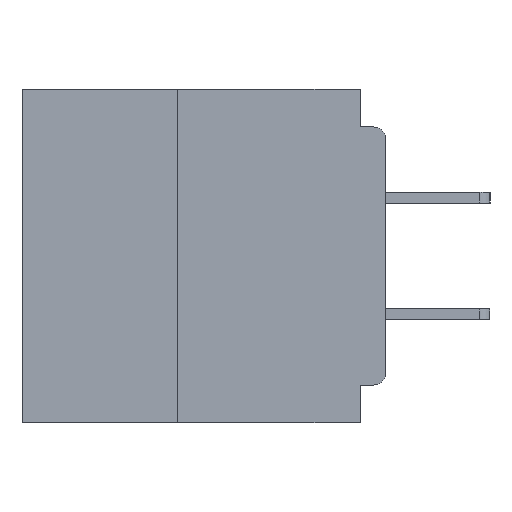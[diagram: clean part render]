
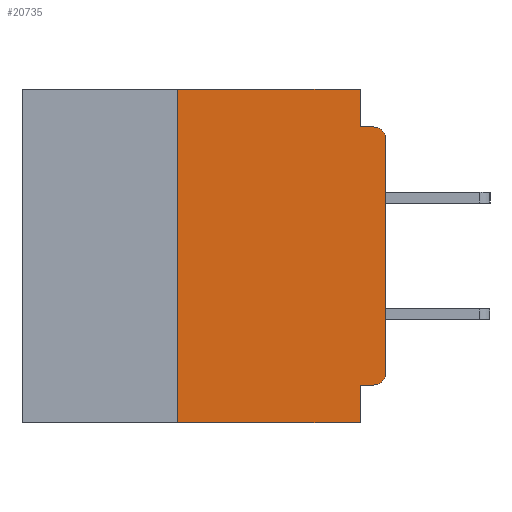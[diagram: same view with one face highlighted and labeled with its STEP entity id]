
A CAD part, left-side view. The second image highlights one B-rep face of the part: STEP entity #20735.
In plain terms, the highlighted planar face has unit normal (-1, 0, 0).
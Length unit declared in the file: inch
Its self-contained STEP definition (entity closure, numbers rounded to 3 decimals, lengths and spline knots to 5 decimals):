
#70 = VECTOR ( 'NONE', #9603, 39.37008 ) ;
#763 = ORIENTED_EDGE ( 'NONE', *, *, #41111, .F. ) ;
#1189 = AXIS2_PLACEMENT_3D ( 'NONE', #9205, #21796, #34524 ) ;
#1302 = ORIENTED_EDGE ( 'NONE', *, *, #34901, .T. ) ;
#3317 = LINE ( 'NONE', #16609, #27731 ) ;
#3838 = CARTESIAN_POINT ( 'NONE',  ( 0., 0.25, -0.4 ) ) ;
#3879 = VERTEX_POINT ( 'NONE', #12400 ) ;
#4194 = DIRECTION ( 'NONE',  ( 0., 0., -1. ) ) ;
#4347 = DIRECTION ( 'NONE',  ( 0., 0., -1. ) ) ;
#4814 = ORIENTED_EDGE ( 'NONE', *, *, #25874, .F. ) ;
#5164 = DIRECTION ( 'NONE',  ( 0., -1., 0. ) ) ;
#6612 = VERTEX_POINT ( 'NONE', #13823 ) ;
#7369 = ORIENTED_EDGE ( 'NONE', *, *, #7548, .T. ) ;
#7548 = EDGE_CURVE ( 'NONE', #29300, #3879, #25821, .T. ) ;
#7783 = VERTEX_POINT ( 'NONE', #19873 ) ;
#8042 = CARTESIAN_POINT ( 'NONE',  ( 0., 0.031, -0.045 ) ) ;
#8632 = CARTESIAN_POINT ( 'NONE',  ( 0., 0.015, -0.045 ) ) ;
#8932 = VECTOR ( 'NONE', #26107, 39.37008 ) ;
#9205 = CARTESIAN_POINT ( 'NONE',  ( 0., 0.437, 0. ) ) ;
#9603 = DIRECTION ( 'NONE',  ( 0., -1., 0. ) ) ;
#10571 = LINE ( 'NONE', #23249, #26465 ) ;
#12393 = PLANE ( 'NONE',  #1189 ) ;
#12400 = CARTESIAN_POINT ( 'NONE',  ( 0., 0., -0.34 ) ) ;
#12407 = LINE ( 'NONE', #19361, #30277 ) ;
#13121 = VERTEX_POINT ( 'NONE', #8042 ) ;
#13267 = VERTEX_POINT ( 'NONE', #15220 ) ;
#13597 = EDGE_CURVE ( 'NONE', #13267, #25910, #10571, .T. ) ;
#13823 = CARTESIAN_POINT ( 'NONE',  ( 0., 0.031, 0. ) ) ;
#13859 = LINE ( 'NONE', #23425, #38057 ) ;
#14188 = LINE ( 'NONE', #21141, #30055 ) ;
#14598 = VECTOR ( 'NONE', #20592, 39.37008 ) ;
#15053 = CARTESIAN_POINT ( 'NONE',  ( 0., 0.031, -0.4 ) ) ;
#15114 = AXIS2_PLACEMENT_3D ( 'NONE', #34560, #15597, #37705 ) ;
#15220 = CARTESIAN_POINT ( 'NONE',  ( 0., 0.031, -0.355 ) ) ;
#15261 = EDGE_CURVE ( 'NONE', #29300, #13267, #12407, .T. ) ;
#15597 = DIRECTION ( 'NONE',  ( -1., 0., 0. ) ) ;
#16156 = VERTEX_POINT ( 'NONE', #26757 ) ;
#16609 = CARTESIAN_POINT ( 'NONE',  ( 0., 0.437, -0.4 ) ) ;
#17343 = LINE ( 'NONE', #3838, #8932 ) ;
#17820 = EDGE_CURVE ( 'NONE', #7783, #25910, #3317, .T. ) ;
#18616 = DIRECTION ( 'NONE',  ( -1., 0., 0. ) ) ;
#19361 = CARTESIAN_POINT ( 'NONE',  ( 0., 0., -0.355 ) ) ;
#19873 = CARTESIAN_POINT ( 'NONE',  ( 0., 0.25, -0.4 ) ) ;
#20253 = ORIENTED_EDGE ( 'NONE', *, *, #13597, .F. ) ;
#20592 = DIRECTION ( 'NONE',  ( 0., 0., 1. ) ) ;
#20735 = ADVANCED_FACE ( 'NONE', ( #21053 ), #12393, .F. ) ;
#20737 = CARTESIAN_POINT ( 'NONE',  ( 0., 0.015, -0.355 ) ) ;
#20836 = EDGE_CURVE ( 'NONE', #13121, #21144, #26544, .T. ) ;
#21053 = FACE_OUTER_BOUND ( 'NONE', #31678, .T. ) ;
#21141 = CARTESIAN_POINT ( 'NONE',  ( 0., 0.437, 0. ) ) ;
#21144 = VERTEX_POINT ( 'NONE', #8632 ) ;
#21796 = DIRECTION ( 'NONE',  ( 1., 0., 0. ) ) ;
#22339 = CARTESIAN_POINT ( 'NONE',  ( 0., 0., -0.045 ) ) ;
#22552 = DIRECTION ( 'NONE',  ( 0., 1., 0. ) ) ;
#23027 = LINE ( 'NONE', #30195, #14598 ) ;
#23249 = CARTESIAN_POINT ( 'NONE',  ( 0., 0.031, -0.4 ) ) ;
#23425 = CARTESIAN_POINT ( 'NONE',  ( 0., 0.031, 0. ) ) ;
#24201 = VERTEX_POINT ( 'NONE', #36608 ) ;
#24225 = ORIENTED_EDGE ( 'NONE', *, *, #20836, .F. ) ;
#24734 = ORIENTED_EDGE ( 'NONE', *, *, #28479, .F. ) ;
#25821 = CIRCLE ( 'NONE', #15114, 0.015 ) ;
#25874 = EDGE_CURVE ( 'NONE', #16156, #6612, #14188, .T. ) ;
#25910 = VERTEX_POINT ( 'NONE', #15053 ) ;
#26107 = DIRECTION ( 'NONE',  ( 0., 0., 1. ) ) ;
#26465 = VECTOR ( 'NONE', #4194, 39.37008 ) ;
#26544 = LINE ( 'NONE', #22339, #70 ) ;
#26757 = CARTESIAN_POINT ( 'NONE',  ( 0., 0.25, 0. ) ) ;
#27731 = VECTOR ( 'NONE', #38717, 39.37008 ) ;
#28479 = EDGE_CURVE ( 'NONE', #7783, #16156, #17343, .T. ) ;
#29300 = VERTEX_POINT ( 'NONE', #20737 ) ;
#30055 = VECTOR ( 'NONE', #5164, 39.37008 ) ;
#30195 = CARTESIAN_POINT ( 'NONE',  ( 0., 0., 0. ) ) ;
#30277 = VECTOR ( 'NONE', #22552, 39.37008 ) ;
#31666 = ORIENTED_EDGE ( 'NONE', *, *, #15261, .F. ) ;
#31678 = EDGE_LOOP ( 'NONE', ( #1302, #34543, #24225, #763, #4814, #24734, #35095, #20253, #31666, #7369 ) ) ;
#31911 = CIRCLE ( 'NONE', #38135, 0.015 ) ;
#34524 = DIRECTION ( 'NONE',  ( 0., 0., -1. ) ) ;
#34543 = ORIENTED_EDGE ( 'NONE', *, *, #35139, .T. ) ;
#34560 = CARTESIAN_POINT ( 'NONE',  ( 0., 0.015, -0.34 ) ) ;
#34901 = EDGE_CURVE ( 'NONE', #3879, #24201, #23027, .T. ) ;
#35095 = ORIENTED_EDGE ( 'NONE', *, *, #17820, .T. ) ;
#35139 = EDGE_CURVE ( 'NONE', #24201, #21144, #31911, .T. ) ;
#36608 = CARTESIAN_POINT ( 'NONE',  ( 0., 0., -0.06 ) ) ;
#37558 = CARTESIAN_POINT ( 'NONE',  ( 0., 0.015, -0.06 ) ) ;
#37705 = DIRECTION ( 'NONE',  ( 0., 0., -1. ) ) ;
#38057 = VECTOR ( 'NONE', #4347, 39.37008 ) ;
#38135 = AXIS2_PLACEMENT_3D ( 'NONE', #37558, #18616, #40730 ) ;
#38717 = DIRECTION ( 'NONE',  ( 0., -1., 0. ) ) ;
#40730 = DIRECTION ( 'NONE',  ( 0., 0., -1. ) ) ;
#41111 = EDGE_CURVE ( 'NONE', #6612, #13121, #13859, .T. ) ;
